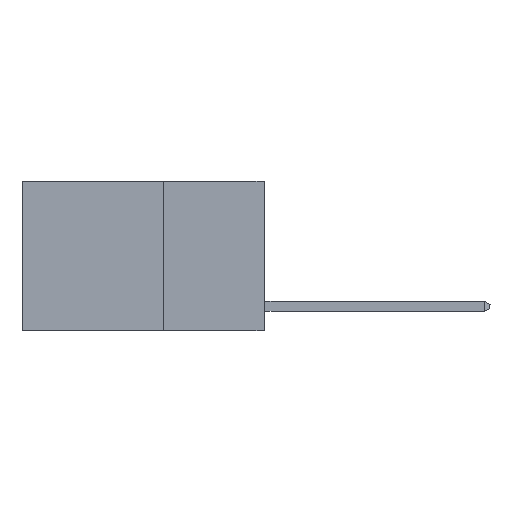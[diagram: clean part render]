
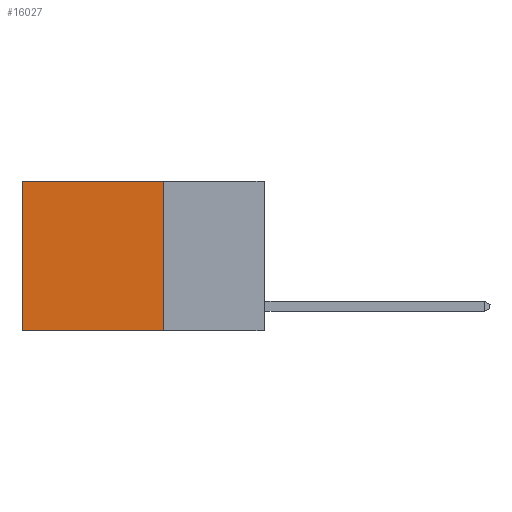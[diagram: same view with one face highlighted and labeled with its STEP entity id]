
A CAD part, left-side view. The second image highlights one B-rep face of the part: STEP entity #16027.
In plain terms, the highlighted planar face has unit normal (-1, 0, 0).
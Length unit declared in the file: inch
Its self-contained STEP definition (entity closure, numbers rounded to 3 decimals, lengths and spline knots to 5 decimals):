
#558 = VERTEX_POINT ( 'NONE', #11242 ) ;
#1260 = AXIS2_PLACEMENT_3D ( 'NONE', #7078, #11777, #3885 ) ;
#1355 = VECTOR ( 'NONE', #13710, 39.37008 ) ;
#2284 = LINE ( 'NONE', #10452, #19466 ) ;
#2696 = CARTESIAN_POINT ( 'NONE',  ( 0.2625, 0.25, -0.37 ) ) ;
#2906 = DIRECTION ( 'NONE',  ( 0., 0., -1. ) ) ;
#3381 = CARTESIAN_POINT ( 'NONE',  ( 0.2625, 0.25, 0. ) ) ;
#3885 = DIRECTION ( 'NONE',  ( 0., 0., -1. ) ) ;
#4430 = ORIENTED_EDGE ( 'NONE', *, *, #7810, .F. ) ;
#5446 = LINE ( 'NONE', #13838, #1355 ) ;
#5543 = LINE ( 'NONE', #2696, #6031 ) ;
#6031 = VECTOR ( 'NONE', #10441, 39.37008 ) ;
#7078 = CARTESIAN_POINT ( 'NONE',  ( 0.2625, 0.25, 0. ) ) ;
#7402 = EDGE_CURVE ( 'NONE', #19444, #17039, #5446, .T. ) ;
#7810 = EDGE_CURVE ( 'NONE', #558, #13447, #2284, .T. ) ;
#10176 = ORIENTED_EDGE ( 'NONE', *, *, #18501, .T. ) ;
#10441 = DIRECTION ( 'NONE',  ( 0., 1., 0. ) ) ;
#10451 = PLANE ( 'NONE',  #1260 ) ;
#10452 = CARTESIAN_POINT ( 'NONE',  ( 0.2625, 0.25, 0. ) ) ;
#11170 = VECTOR ( 'NONE', #17199, 39.37008 ) ;
#11242 = CARTESIAN_POINT ( 'NONE',  ( 0.2625, 0.25, 0. ) ) ;
#11777 = DIRECTION ( 'NONE',  ( 1., 0., 0. ) ) ;
#13447 = VERTEX_POINT ( 'NONE', #19467 ) ;
#13545 = CARTESIAN_POINT ( 'NONE',  ( 0.2625, 0.6, 0. ) ) ;
#13710 = DIRECTION ( 'NONE',  ( 0., 0., -1. ) ) ;
#13838 = CARTESIAN_POINT ( 'NONE',  ( 0.2625, 0.6, 0. ) ) ;
#15645 = FACE_OUTER_BOUND ( 'NONE', #19931, .T. ) ;
#15793 = LINE ( 'NONE', #3381, #11170 ) ;
#16027 = ADVANCED_FACE ( 'NONE', ( #15645 ), #10451, .F. ) ;
#16542 = ORIENTED_EDGE ( 'NONE', *, *, #7402, .T. ) ;
#16842 = CARTESIAN_POINT ( 'NONE',  ( 0.2625, 0.6, -0.37 ) ) ;
#17039 = VERTEX_POINT ( 'NONE', #16842 ) ;
#17199 = DIRECTION ( 'NONE',  ( 0., 1., 0. ) ) ;
#17659 = ORIENTED_EDGE ( 'NONE', *, *, #19790, .F. ) ;
#18501 = EDGE_CURVE ( 'NONE', #558, #19444, #15793, .T. ) ;
#19444 = VERTEX_POINT ( 'NONE', #13545 ) ;
#19466 = VECTOR ( 'NONE', #2906, 39.37008 ) ;
#19467 = CARTESIAN_POINT ( 'NONE',  ( 0.2625, 0.25, -0.37 ) ) ;
#19790 = EDGE_CURVE ( 'NONE', #13447, #17039, #5543, .T. ) ;
#19931 = EDGE_LOOP ( 'NONE', ( #16542, #17659, #4430, #10176 ) ) ;
